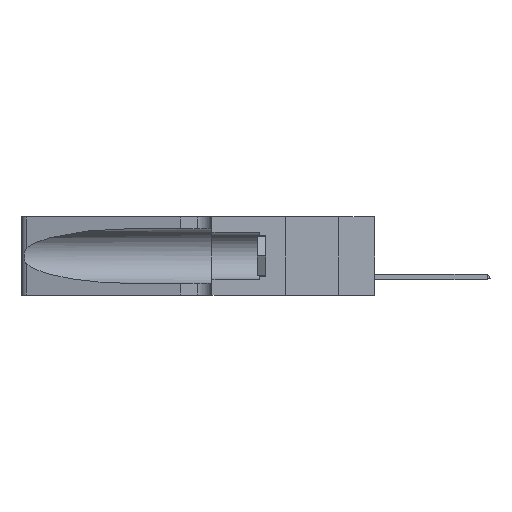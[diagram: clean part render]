
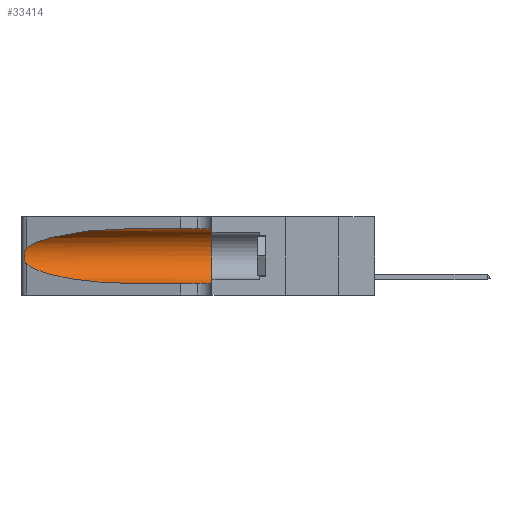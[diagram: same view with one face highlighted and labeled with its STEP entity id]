
A CAD part, left-side view. The second image highlights one B-rep face of the part: STEP entity #33414.
In plain terms, the highlighted cylindrical face has radius 3.308 mm (diameter 6.617 mm), a partial arc.
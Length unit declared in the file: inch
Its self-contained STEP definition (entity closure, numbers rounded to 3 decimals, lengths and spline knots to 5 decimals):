
#109 = CARTESIAN_POINT ( 'NONE',  ( 0.1305, 0.72297, 0.05475 ) ) ;
#351 = VERTEX_POINT ( 'NONE', #27396 ) ;
#801 = CARTESIAN_POINT ( 'NONE',  ( 0.25555, 1.22993, 0.14849 ) ) ;
#2022 = CARTESIAN_POINT ( 'NONE',  ( 0.1305, 1.61858, 0.185 ) ) ;
#2987 = CARTESIAN_POINT ( 'NONE',  ( 0.25487, 1.22718, 0.22369 ) ) ;
#3038 = DIRECTION ( 'NONE',  ( 0., -1., 0. ) ) ;
#3061 = DIRECTION ( 'NONE',  ( 0., -1., 0. ) ) ;
#3208 = AXIS2_PLACEMENT_3D ( 'NONE', #22600, #13707, #37284 ) ;
#3634 = CIRCLE ( 'NONE', #3208, 0.13025 ) ;
#4744 = EDGE_CURVE ( 'NONE', #30887, #11669, #20133, .T. ) ;
#6115 = CARTESIAN_POINT ( 'NONE',  ( 0.25854, 1.2359, 0.20912 ) ) ;
#6658 = FACE_OUTER_BOUND ( 'NONE', #20751, .T. ) ;
#6812 = VERTEX_POINT ( 'NONE', #38519 ) ;
#6822 = EDGE_CURVE ( 'NONE', #11669, #6812, #37235, .T. ) ;
#6971 = VERTEX_POINT ( 'NONE', #14857 ) ;
#8389 = LINE ( 'NONE', #21507, #15848 ) ;
#8574 = CARTESIAN_POINT ( 'NONE',  ( 0.18966, 0.96281, 0.05475 ) ) ;
#9035 = CARTESIAN_POINT ( 'NONE',  ( 0.25856, 1.23593, 0.16098 ) ) ;
#11669 = VERTEX_POINT ( 'NONE', #36707 ) ;
#11831 = CARTESIAN_POINT ( 'NONE',  ( 0.25787, 1.23484, 0.2124 ) ) ;
#11956 = CARTESIAN_POINT ( 'NONE',  ( 0.26018, 1.23835, 0.19895 ) ) ;
#13108 = B_SPLINE_CURVE_WITH_KNOTS ( 'NONE', 3,
 ( #2987, #36073, #23755, #11831, #6115, #11956, #23994, #18100, #26991, #9035, #21109, #34187, #801, #34743 ),
 .UNSPECIFIED., .F., .F.,
 ( 4, 2, 2, 2, 2, 2, 4 ),
 ( 0., 0.00027, 0.00053, 0.00107, 0.0016, 0.00187, 0.00214 ),
 .UNSPECIFIED. ) ;
#13707 = DIRECTION ( 'NONE',  ( 0., 1., 0. ) ) ;
#14857 = CARTESIAN_POINT ( 'NONE',  ( 0.1305, 0.72297, 0.31525 ) ) ;
#15526 = ORIENTED_EDGE ( 'NONE', *, *, #6822, .T. ) ;
#15848 = VECTOR ( 'NONE', #3038, 39.37008 ) ;
#16183 = EDGE_CURVE ( 'NONE', #21057, #30887, #13108, .T. ) ;
#16381 = ORIENTED_EDGE ( 'NONE', *, *, #19748, .F. ) ;
#16420 = ORIENTED_EDGE ( 'NONE', *, *, #28553, .T. ) ;
#18100 = CARTESIAN_POINT ( 'NONE',  ( 0.26075, 1.23896, 0.178 ) ) ;
#18131 = CARTESIAN_POINT ( 'NONE',  ( 0.1305, 1.61858, 0.05475 ) ) ;
#19748 = EDGE_CURVE ( 'NONE', #6971, #351, #8389, .T. ) ;
#20133 =( BOUNDED_CURVE ( )  B_SPLINE_CURVE ( 3, ( #23779, #35487, #8574, #109 ),
 .UNSPECIFIED., .F., .T. ) 
 B_SPLINE_CURVE_WITH_KNOTS ( ( 4, 4 ),
 ( 3.44316, 4.71239 ),
 .UNSPECIFIED. ) 
 CURVE ( )  GEOMETRIC_REPRESENTATION_ITEM ( )  RATIONAL_B_SPLINE_CURVE ( ( 1., 0.87, 0.87, 1. ) ) 
 REPRESENTATION_ITEM ( '' )  );
#20751 = EDGE_LOOP ( 'NONE', ( #16420, #24809, #26707, #15526, #36723, #16381 ) ) ;
#21057 = VERTEX_POINT ( 'NONE', #32971 ) ;
#21109 = CARTESIAN_POINT ( 'NONE',  ( 0.25789, 1.23486, 0.15765 ) ) ;
#21507 = CARTESIAN_POINT ( 'NONE',  ( 0.1305, 1.61858, 0.31525 ) ) ;
#22600 = CARTESIAN_POINT ( 'NONE',  ( 0.1305, 0.35, 0.185 ) ) ;
#23755 = CARTESIAN_POINT ( 'NONE',  ( 0.25639, 1.23184, 0.21858 ) ) ;
#23779 = CARTESIAN_POINT ( 'NONE',  ( 0.25487, 1.22718, 0.14631 ) ) ;
#23994 = CARTESIAN_POINT ( 'NONE',  ( 0.26075, 1.23896, 0.19203 ) ) ;
#24148 =( BOUNDED_CURVE ( )  B_SPLINE_CURVE ( 3, ( #28914, #32031, #35077, #38452 ),
 .UNSPECIFIED., .F., .F. ) 
 B_SPLINE_CURVE_WITH_KNOTS ( ( 4, 4 ),
 ( 1.5708, 2.84003 ),
 .UNSPECIFIED. ) 
 CURVE ( )  GEOMETRIC_REPRESENTATION_ITEM ( )  RATIONAL_B_SPLINE_CURVE ( ( 1., 0.87, 0.87, 1. ) ) 
 REPRESENTATION_ITEM ( '' )  );
#24809 = ORIENTED_EDGE ( 'NONE', *, *, #16183, .T. ) ;
#25597 = EDGE_CURVE ( 'NONE', #351, #6812, #3634, .T. ) ;
#26707 = ORIENTED_EDGE ( 'NONE', *, *, #4744, .T. ) ;
#26991 = CARTESIAN_POINT ( 'NONE',  ( 0.26017, 1.23833, 0.17102 ) ) ;
#27396 = CARTESIAN_POINT ( 'NONE',  ( 0.1305, 0.35, 0.31525 ) ) ;
#28553 = EDGE_CURVE ( 'NONE', #6971, #21057, #24148, .T. ) ;
#28914 = CARTESIAN_POINT ( 'NONE',  ( 0.1305, 0.72297, 0.31525 ) ) ;
#29236 = CARTESIAN_POINT ( 'NONE',  ( 0.25487, 1.22718, 0.14631 ) ) ;
#30887 = VERTEX_POINT ( 'NONE', #29236 ) ;
#31786 = DIRECTION ( 'NONE',  ( 0., -1., 0. ) ) ;
#32031 = CARTESIAN_POINT ( 'NONE',  ( 0.18966, 0.96281, 0.31525 ) ) ;
#32101 = CYLINDRICAL_SURFACE ( 'NONE', #34356, 0.13025 ) ;
#32971 = CARTESIAN_POINT ( 'NONE',  ( 0.25487, 1.22718, 0.22369 ) ) ;
#33414 = ADVANCED_FACE ( 'NONE', ( #6658 ), #32101, .F. ) ;
#34187 = CARTESIAN_POINT ( 'NONE',  ( 0.25639, 1.23186, 0.15144 ) ) ;
#34356 = AXIS2_PLACEMENT_3D ( 'NONE', #2022, #31786, #37716 ) ;
#34423 = VECTOR ( 'NONE', #3061, 39.37008 ) ;
#34743 = CARTESIAN_POINT ( 'NONE',  ( 0.25487, 1.22718, 0.14631 ) ) ;
#35077 = CARTESIAN_POINT ( 'NONE',  ( 0.2373, 1.15595, 0.28018 ) ) ;
#35487 = CARTESIAN_POINT ( 'NONE',  ( 0.2373, 1.15595, 0.08982 ) ) ;
#36073 = CARTESIAN_POINT ( 'NONE',  ( 0.25555, 1.22994, 0.2215 ) ) ;
#36707 = CARTESIAN_POINT ( 'NONE',  ( 0.1305, 0.72297, 0.05475 ) ) ;
#36723 = ORIENTED_EDGE ( 'NONE', *, *, #25597, .F. ) ;
#37235 = LINE ( 'NONE', #18131, #34423 ) ;
#37284 = DIRECTION ( 'NONE',  ( 0., 0., 1. ) ) ;
#37716 = DIRECTION ( 'NONE',  ( 0., 0., -1. ) ) ;
#38452 = CARTESIAN_POINT ( 'NONE',  ( 0.25487, 1.22718, 0.22369 ) ) ;
#38519 = CARTESIAN_POINT ( 'NONE',  ( 0.1305, 0.35, 0.05475 ) ) ;
